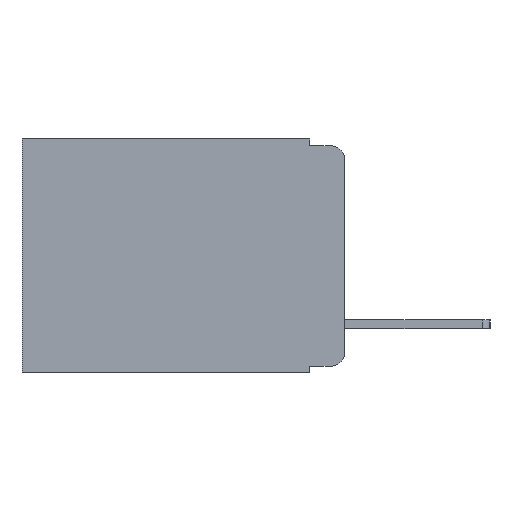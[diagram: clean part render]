
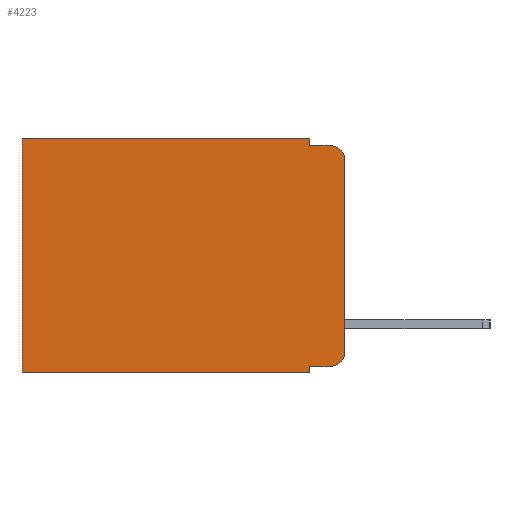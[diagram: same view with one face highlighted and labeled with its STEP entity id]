
A CAD part, left-side view. The second image highlights one B-rep face of the part: STEP entity #4223.
In plain terms, the highlighted planar face has unit normal (-1, 0, 0).
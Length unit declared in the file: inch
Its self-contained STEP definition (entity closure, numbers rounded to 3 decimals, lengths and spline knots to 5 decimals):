
#434 = ORIENTED_EDGE ( 'NONE', *, *, #2754, .F. ) ;
#494 = FACE_OUTER_BOUND ( 'NONE', #3322, .T. ) ;
#531 = CARTESIAN_POINT ( 'NONE',  ( 0.298, 0.02, -0.01 ) ) ;
#597 = EDGE_CURVE ( 'NONE', #9118, #7478, #6050, .T. ) ;
#674 = CARTESIAN_POINT ( 'NONE',  ( 0.298, 0.051, 0. ) ) ;
#929 = CARTESIAN_POINT ( 'NONE',  ( 0.298, 0.473, 0. ) ) ;
#1057 = ORIENTED_EDGE ( 'NONE', *, *, #1862, .T. ) ;
#1353 = LINE ( 'NONE', #5499, #10111 ) ;
#1369 = CIRCLE ( 'NONE', #2858, 0.02 ) ;
#1444 = CARTESIAN_POINT ( 'NONE',  ( 0.298, 0.02, -0.03 ) ) ;
#1567 = CARTESIAN_POINT ( 'NONE',  ( 0.298, 0., 0. ) ) ;
#1654 = EDGE_CURVE ( 'NONE', #2735, #5834, #3649, .T. ) ;
#1862 = EDGE_CURVE ( 'NONE', #5070, #9723, #7921, .T. ) ;
#1910 = CARTESIAN_POINT ( 'NONE',  ( 0.298, 0.473, 0. ) ) ;
#1986 = DIRECTION ( 'NONE',  ( 0., 0., -1. ) ) ;
#2297 = EDGE_CURVE ( 'NONE', #10022, #5834, #1369, .T. ) ;
#2483 = ORIENTED_EDGE ( 'NONE', *, *, #1654, .F. ) ;
#2639 = CARTESIAN_POINT ( 'NONE',  ( 0.298, 0.473, -0.343 ) ) ;
#2683 = CARTESIAN_POINT ( 'NONE',  ( 0.298, 0.051, -0.01 ) ) ;
#2735 = VERTEX_POINT ( 'NONE', #3747 ) ;
#2754 = EDGE_CURVE ( 'NONE', #10022, #7478, #10117, .T. ) ;
#2783 = LINE ( 'NONE', #5056, #3328 ) ;
#2834 = DIRECTION ( 'NONE',  ( 0., -1., 0. ) ) ;
#2858 = AXIS2_PLACEMENT_3D ( 'NONE', #1444, #10590, #6924 ) ;
#2995 = ORIENTED_EDGE ( 'NONE', *, *, #5865, .T. ) ;
#3081 = CARTESIAN_POINT ( 'NONE',  ( 0.298, 0.051, 0. ) ) ;
#3230 = EDGE_CURVE ( 'NONE', #5280, #7597, #10106, .T. ) ;
#3272 = DIRECTION ( 'NONE',  ( 0., 0., -1. ) ) ;
#3322 = EDGE_LOOP ( 'NONE', ( #434, #3580, #2483, #4018, #6097, #1057, #9657, #10074, #2995, #5426 ) ) ;
#3328 = VECTOR ( 'NONE', #10917, 39.37008 ) ;
#3402 = VECTOR ( 'NONE', #7861, 39.37008 ) ;
#3569 = CARTESIAN_POINT ( 'NONE',  ( 0.298, 0., 0. ) ) ;
#3580 = ORIENTED_EDGE ( 'NONE', *, *, #2297, .T. ) ;
#3621 = LINE ( 'NONE', #3569, #10100 ) ;
#3634 = DIRECTION ( 'NONE',  ( 0., 1., 0. ) ) ;
#3649 = LINE ( 'NONE', #2683, #9879 ) ;
#3747 = CARTESIAN_POINT ( 'NONE',  ( 0.298, 0.051, -0.01 ) ) ;
#4018 = ORIENTED_EDGE ( 'NONE', *, *, #8103, .F. ) ;
#4223 = ADVANCED_FACE ( 'NONE', ( #494 ), #9773, .F. ) ;
#4244 = DIRECTION ( 'NONE',  ( 0., -1., 0. ) ) ;
#4653 = DIRECTION ( 'NONE',  ( -1., 0., 0. ) ) ;
#4860 = CARTESIAN_POINT ( 'NONE',  ( 0.298, 0.051, -0.333 ) ) ;
#5056 = CARTESIAN_POINT ( 'NONE',  ( 0.298, 0., -0.343 ) ) ;
#5070 = VERTEX_POINT ( 'NONE', #929 ) ;
#5280 = VERTEX_POINT ( 'NONE', #6366 ) ;
#5426 = ORIENTED_EDGE ( 'NONE', *, *, #597, .T. ) ;
#5499 = CARTESIAN_POINT ( 'NONE',  ( 0.298, 0.051, 0. ) ) ;
#5748 = DIRECTION ( 'NONE',  ( 0., 0., -1. ) ) ;
#5834 = VERTEX_POINT ( 'NONE', #531 ) ;
#5865 = EDGE_CURVE ( 'NONE', #5280, #9118, #10413, .T. ) ;
#6050 = CIRCLE ( 'NONE', #8494, 0.02 ) ;
#6097 = ORIENTED_EDGE ( 'NONE', *, *, #8603, .T. ) ;
#6366 = CARTESIAN_POINT ( 'NONE',  ( 0.298, 0.051, -0.333 ) ) ;
#6924 = DIRECTION ( 'NONE',  ( 0., 0., -1. ) ) ;
#7305 = CARTESIAN_POINT ( 'NONE',  ( 0.298, 0.02, -0.333 ) ) ;
#7478 = VERTEX_POINT ( 'NONE', #10205 ) ;
#7597 = VERTEX_POINT ( 'NONE', #8607 ) ;
#7861 = DIRECTION ( 'NONE',  ( 0., 0., -1. ) ) ;
#7885 = VECTOR ( 'NONE', #3272, 39.37008 ) ;
#7921 = LINE ( 'NONE', #1910, #3402 ) ;
#7933 = VECTOR ( 'NONE', #4244, 39.37008 ) ;
#8103 = EDGE_CURVE ( 'NONE', #10587, #2735, #1353, .T. ) ;
#8227 = DIRECTION ( 'NONE',  ( 0., 0., -1. ) ) ;
#8334 = CARTESIAN_POINT ( 'NONE',  ( 0.298, 0., 0. ) ) ;
#8438 = AXIS2_PLACEMENT_3D ( 'NONE', #8334, #10709, #10689 ) ;
#8494 = AXIS2_PLACEMENT_3D ( 'NONE', #10403, #4653, #5748 ) ;
#8603 = EDGE_CURVE ( 'NONE', #10587, #5070, #3621, .T. ) ;
#8607 = CARTESIAN_POINT ( 'NONE',  ( 0.298, 0.051, -0.343 ) ) ;
#9118 = VERTEX_POINT ( 'NONE', #7305 ) ;
#9589 = EDGE_CURVE ( 'NONE', #7597, #9723, #2783, .T. ) ;
#9657 = ORIENTED_EDGE ( 'NONE', *, *, #9589, .F. ) ;
#9723 = VERTEX_POINT ( 'NONE', #2639 ) ;
#9765 = CARTESIAN_POINT ( 'NONE',  ( 0.298, 0., -0.03 ) ) ;
#9773 = PLANE ( 'NONE',  #8438 ) ;
#9879 = VECTOR ( 'NONE', #2834, 39.37008 ) ;
#10022 = VERTEX_POINT ( 'NONE', #9765 ) ;
#10074 = ORIENTED_EDGE ( 'NONE', *, *, #3230, .F. ) ;
#10100 = VECTOR ( 'NONE', #3634, 39.37008 ) ;
#10106 = LINE ( 'NONE', #674, #7885 ) ;
#10111 = VECTOR ( 'NONE', #1986, 39.37008 ) ;
#10117 = LINE ( 'NONE', #1567, #10377 ) ;
#10205 = CARTESIAN_POINT ( 'NONE',  ( 0.298, 0., -0.313 ) ) ;
#10377 = VECTOR ( 'NONE', #8227, 39.37008 ) ;
#10403 = CARTESIAN_POINT ( 'NONE',  ( 0.298, 0.02, -0.313 ) ) ;
#10413 = LINE ( 'NONE', #4860, #7933 ) ;
#10587 = VERTEX_POINT ( 'NONE', #3081 ) ;
#10590 = DIRECTION ( 'NONE',  ( -1., 0., 0. ) ) ;
#10689 = DIRECTION ( 'NONE',  ( 0., 0., -1. ) ) ;
#10709 = DIRECTION ( 'NONE',  ( 1., 0., 0. ) ) ;
#10917 = DIRECTION ( 'NONE',  ( 0., 1., 0. ) ) ;
